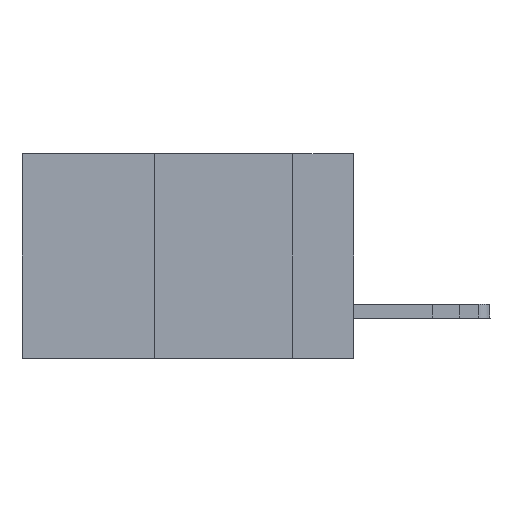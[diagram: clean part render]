
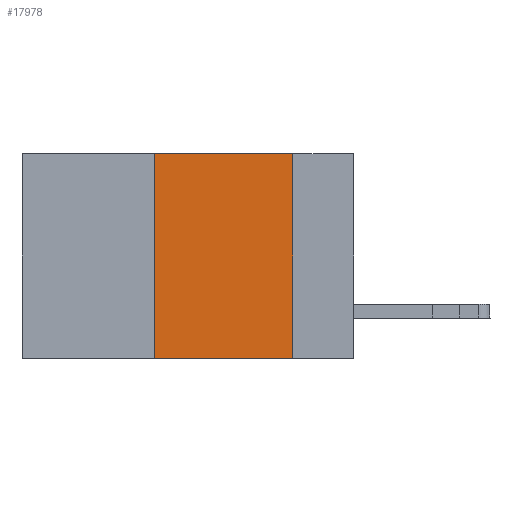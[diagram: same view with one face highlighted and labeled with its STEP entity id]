
A CAD part, left-side view. The second image highlights one B-rep face of the part: STEP entity #17978.
In plain terms, the highlighted planar face has unit normal (-1, 0, 0).
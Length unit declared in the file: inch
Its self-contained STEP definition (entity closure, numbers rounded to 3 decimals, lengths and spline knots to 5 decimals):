
#306 = VECTOR ( 'NONE', #2388, 39.37008 ) ;
#581 = EDGE_CURVE ( 'NONE', #13571, #9105, #17990, .T. ) ;
#1009 = ORIENTED_EDGE ( 'NONE', *, *, #24124, .F. ) ;
#1560 = EDGE_CURVE ( 'NONE', #21905, #9105, #10189, .T. ) ;
#1719 = VECTOR ( 'NONE', #18135, 39.37008 ) ;
#2388 = DIRECTION ( 'NONE',  ( 0., 0., 1. ) ) ;
#2432 = VECTOR ( 'NONE', #20001, 39.37008 ) ;
#2874 = CARTESIAN_POINT ( 'NONE',  ( 0., 0.36, -0.37 ) ) ;
#4575 = DIRECTION ( 'NONE',  ( 1., 0., 0. ) ) ;
#5219 = EDGE_LOOP ( 'NONE', ( #19904, #12427, #1009, #8610 ) ) ;
#6769 = CARTESIAN_POINT ( 'NONE',  ( 0., 0.6, -0.37 ) ) ;
#8586 = FACE_OUTER_BOUND ( 'NONE', #5219, .T. ) ;
#8610 = ORIENTED_EDGE ( 'NONE', *, *, #581, .T. ) ;
#8844 = CARTESIAN_POINT ( 'NONE',  ( 0., 0.6, 0. ) ) ;
#9105 = VERTEX_POINT ( 'NONE', #17060 ) ;
#10164 = CARTESIAN_POINT ( 'NONE',  ( 0., 0.36, 0. ) ) ;
#10189 = LINE ( 'NONE', #23539, #1719 ) ;
#10943 = CARTESIAN_POINT ( 'NONE',  ( 0., 0.36, 0. ) ) ;
#12427 = ORIENTED_EDGE ( 'NONE', *, *, #15301, .F. ) ;
#13571 = VERTEX_POINT ( 'NONE', #2874 ) ;
#15301 = EDGE_CURVE ( 'NONE', #17400, #21905, #22852, .T. ) ;
#16286 = DIRECTION ( 'NONE',  ( 0., 0., -1. ) ) ;
#17060 = CARTESIAN_POINT ( 'NONE',  ( 0., 0.11, -0.37 ) ) ;
#17400 = VERTEX_POINT ( 'NONE', #10943 ) ;
#17867 = VECTOR ( 'NONE', #20478, 39.37008 ) ;
#17978 = ADVANCED_FACE ( 'NONE', ( #8586 ), #24071, .F. ) ;
#17990 = LINE ( 'NONE', #6769, #2432 ) ;
#18135 = DIRECTION ( 'NONE',  ( 0., 0., -1. ) ) ;
#18704 = CARTESIAN_POINT ( 'NONE',  ( 0., 0.6, 0. ) ) ;
#19904 = ORIENTED_EDGE ( 'NONE', *, *, #1560, .F. ) ;
#20001 = DIRECTION ( 'NONE',  ( 0., -1., 0. ) ) ;
#20478 = DIRECTION ( 'NONE',  ( 0., -1., 0. ) ) ;
#21905 = VERTEX_POINT ( 'NONE', #22949 ) ;
#22401 = AXIS2_PLACEMENT_3D ( 'NONE', #8844, #4575, #16286 ) ;
#22632 = LINE ( 'NONE', #10164, #306 ) ;
#22852 = LINE ( 'NONE', #18704, #17867 ) ;
#22949 = CARTESIAN_POINT ( 'NONE',  ( 0., 0.11, 0. ) ) ;
#23539 = CARTESIAN_POINT ( 'NONE',  ( 0., 0.11, 0. ) ) ;
#24071 = PLANE ( 'NONE',  #22401 ) ;
#24124 = EDGE_CURVE ( 'NONE', #13571, #17400, #22632, .T. ) ;
